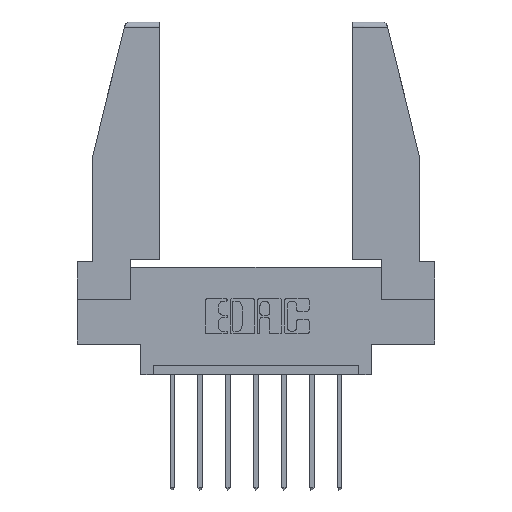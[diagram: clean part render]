
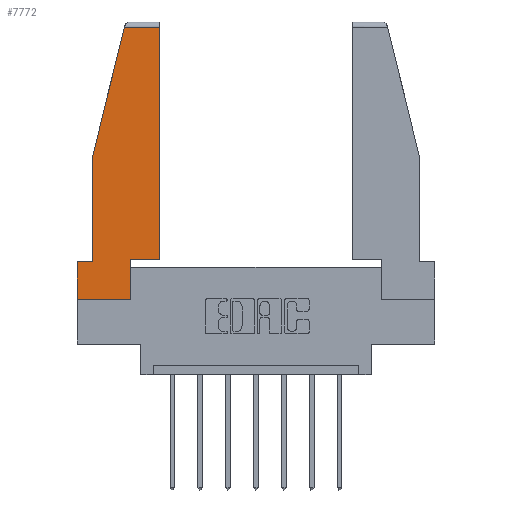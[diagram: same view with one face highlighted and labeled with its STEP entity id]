
A CAD part, top view. The second image highlights one B-rep face of the part: STEP entity #7772.
In plain terms, the highlighted planar face has unit normal (0, 0, 1).
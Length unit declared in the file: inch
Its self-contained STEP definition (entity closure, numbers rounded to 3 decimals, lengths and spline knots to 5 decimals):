
#15 = CARTESIAN_POINT ( 'NONE',  ( 0., 0., 0. ) ) ;
#354 = DIRECTION ( 'NONE',  ( 0., 1., 0. ) ) ;
#593 = CARTESIAN_POINT ( 'NONE',  ( 0.086, 0.8, 0. ) ) ;
#986 = DIRECTION ( 'NONE',  ( 0., -1., 0. ) ) ;
#1095 = EDGE_LOOP ( 'NONE', ( #10628, #2041, #1303, #7382, #4332, #3297, #5520, #4179, #7284 ) ) ;
#1303 = ORIENTED_EDGE ( 'NONE', *, *, #2639, .T. ) ;
#1349 = CARTESIAN_POINT ( 'NONE',  ( 0.461, 1.52, 0. ) ) ;
#1425 = CARTESIAN_POINT ( 'NONE',  ( 0.297, 0., 0. ) ) ;
#1486 = CARTESIAN_POINT ( 'NONE',  ( 0.086, 0.8, 0. ) ) ;
#1781 = PLANE ( 'NONE',  #7623 ) ;
#1893 = DIRECTION ( 'NONE',  ( 0., 0., 1. ) ) ;
#2041 = ORIENTED_EDGE ( 'NONE', *, *, #10763, .T. ) ;
#2047 = LINE ( 'NONE', #7981, #10443 ) ;
#2287 = VERTEX_POINT ( 'NONE', #1425 ) ;
#2504 = DIRECTION ( 'NONE',  ( 0., 1., 0. ) ) ;
#2639 = EDGE_CURVE ( 'NONE', #2769, #11687, #4173, .T. ) ;
#2735 = EDGE_CURVE ( 'NONE', #10375, #6816, #4476, .T. ) ;
#2769 = VERTEX_POINT ( 'NONE', #10381 ) ;
#2808 = CARTESIAN_POINT ( 'NONE',  ( 0., 0.21, 0. ) ) ;
#2857 = VERTEX_POINT ( 'NONE', #4523 ) ;
#2881 = FACE_OUTER_BOUND ( 'NONE', #1095, .T. ) ;
#2964 = LINE ( 'NONE', #8213, #6378 ) ;
#2984 = CARTESIAN_POINT ( 'NONE',  ( 0.086, 0.21, 0. ) ) ;
#3080 = VERTEX_POINT ( 'NONE', #5629 ) ;
#3251 = CARTESIAN_POINT ( 'NONE',  ( 0.461, 0.223, 0. ) ) ;
#3297 = ORIENTED_EDGE ( 'NONE', *, *, #6499, .T. ) ;
#3385 = LINE ( 'NONE', #2808, #10429 ) ;
#4126 = LINE ( 'NONE', #6434, #10153 ) ;
#4173 = LINE ( 'NONE', #11839, #10338 ) ;
#4179 = ORIENTED_EDGE ( 'NONE', *, *, #4293, .T. ) ;
#4293 = EDGE_CURVE ( 'NONE', #2287, #10375, #2964, .T. ) ;
#4332 = ORIENTED_EDGE ( 'NONE', *, *, #5623, .T. ) ;
#4476 = LINE ( 'NONE', #7585, #11961 ) ;
#4523 = CARTESIAN_POINT ( 'NONE',  ( 0., 0., 0. ) ) ;
#5191 = EDGE_CURVE ( 'NONE', #2857, #2287, #4126, .T. ) ;
#5230 = DIRECTION ( 'NONE',  ( 0., -1., 0. ) ) ;
#5520 = ORIENTED_EDGE ( 'NONE', *, *, #5191, .T. ) ;
#5623 = EDGE_CURVE ( 'NONE', #9277, #3080, #3385, .T. ) ;
#5629 = CARTESIAN_POINT ( 'NONE',  ( 0., 0.21, 0. ) ) ;
#6327 = VECTOR ( 'NONE', #5230, 39.37008 ) ;
#6378 = VECTOR ( 'NONE', #2504, 39.37008 ) ;
#6434 = CARTESIAN_POINT ( 'NONE',  ( 0., 0., 0. ) ) ;
#6471 = VECTOR ( 'NONE', #986, 39.37008 ) ;
#6499 = EDGE_CURVE ( 'NONE', #3080, #2857, #9013, .T. ) ;
#6816 = VERTEX_POINT ( 'NONE', #9657 ) ;
#6978 = VECTOR ( 'NONE', #354, 39.37008 ) ;
#7284 = ORIENTED_EDGE ( 'NONE', *, *, #2735, .T. ) ;
#7382 = ORIENTED_EDGE ( 'NONE', *, *, #12099, .T. ) ;
#7470 = DIRECTION ( 'NONE',  ( -1., 0., 0. ) ) ;
#7503 = DIRECTION ( 'NONE',  ( 1., 0., 0. ) ) ;
#7585 = CARTESIAN_POINT ( 'NONE',  ( 0.297, 0.223, 0. ) ) ;
#7623 = AXIS2_PLACEMENT_3D ( 'NONE', #15, #1893, #8438 ) ;
#7768 = DIRECTION ( 'NONE',  ( 1., 0., 0. ) ) ;
#7772 = ADVANCED_FACE ( 'NONE', ( #2881 ), #1781, .T. ) ;
#7981 = CARTESIAN_POINT ( 'NONE',  ( 0., 1.52, 0. ) ) ;
#8194 = LINE ( 'NONE', #3251, #6978 ) ;
#8213 = CARTESIAN_POINT ( 'NONE',  ( 0.297, 0., 0. ) ) ;
#8438 = DIRECTION ( 'NONE',  ( 1., 0., 0. ) ) ;
#8714 = EDGE_CURVE ( 'NONE', #6816, #9876, #8194, .T. ) ;
#8871 = LINE ( 'NONE', #593, #6327 ) ;
#8966 = DIRECTION ( 'NONE',  ( -0.239, -0.971, 0. ) ) ;
#9013 = LINE ( 'NONE', #9586, #6471 ) ;
#9277 = VERTEX_POINT ( 'NONE', #2984 ) ;
#9586 = CARTESIAN_POINT ( 'NONE',  ( 0., 0.21, 0. ) ) ;
#9657 = CARTESIAN_POINT ( 'NONE',  ( 0.461, 0.223, 0. ) ) ;
#9876 = VERTEX_POINT ( 'NONE', #1349 ) ;
#10153 = VECTOR ( 'NONE', #7768, 39.37008 ) ;
#10338 = VECTOR ( 'NONE', #8966, 39.37008 ) ;
#10375 = VERTEX_POINT ( 'NONE', #10774 ) ;
#10381 = CARTESIAN_POINT ( 'NONE',  ( 0.2636, 1.52, 0. ) ) ;
#10429 = VECTOR ( 'NONE', #7470, 39.37008 ) ;
#10443 = VECTOR ( 'NONE', #10822, 39.37008 ) ;
#10628 = ORIENTED_EDGE ( 'NONE', *, *, #8714, .T. ) ;
#10763 = EDGE_CURVE ( 'NONE', #9876, #2769, #2047, .T. ) ;
#10774 = CARTESIAN_POINT ( 'NONE',  ( 0.297, 0.223, 0. ) ) ;
#10822 = DIRECTION ( 'NONE',  ( -1., 0., 0. ) ) ;
#11687 = VERTEX_POINT ( 'NONE', #1486 ) ;
#11839 = CARTESIAN_POINT ( 'NONE',  ( 0.271, 1.55, 0. ) ) ;
#11961 = VECTOR ( 'NONE', #7503, 39.37008 ) ;
#12099 = EDGE_CURVE ( 'NONE', #11687, #9277, #8871, .T. ) ;
